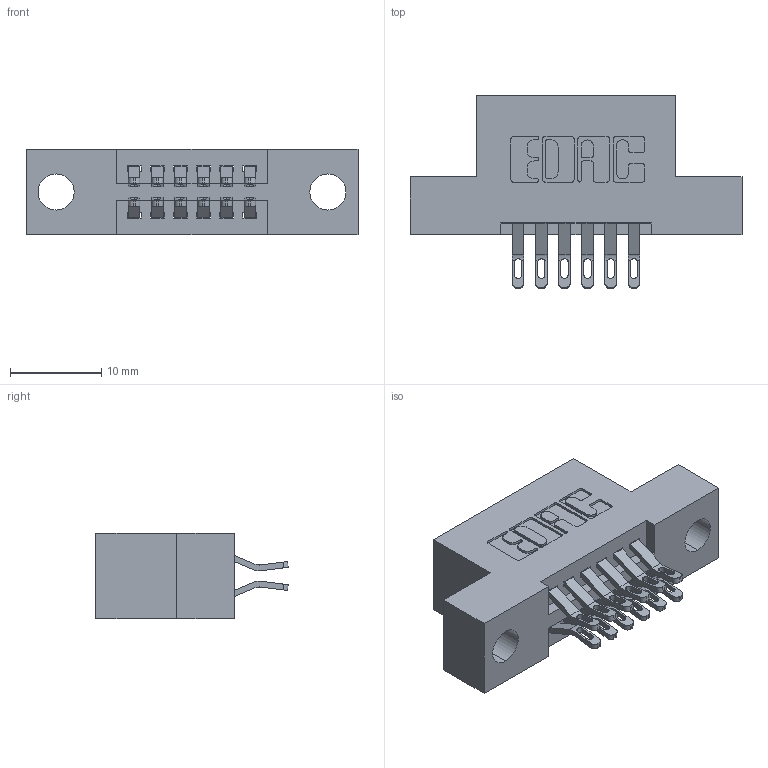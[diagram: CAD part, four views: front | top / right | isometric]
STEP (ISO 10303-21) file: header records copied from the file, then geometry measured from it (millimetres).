
FILE_DESCRIPTION (( 'STEP AP203' ), '1' );
FILE_NAME ('345-012-555-204.STEP', '2021-05-19T15:48:22', ( '' ), ( '' ), 'SwSTEP 2.0', 'SolidWorks 2020', '' );
FILE_SCHEMA (( 'CONFIG_CONTROL_DESIGN' ));
Length unit declared in the file: inch
Products named in the file (3): 345-012-555-204; 345-292-001_555 Tail; 345 Part_Flush Mounting Lugs - 0.156 Dia-TI
Assembly tree (13 placements, depth 2):
  345-012-555-204
    345 Part_Flush Mounting Lugs - 0.156 Dia-TI
    345-292-001_555 Tail  x12
Bounding box: 36.45 x 21.13 x 9.4 mm (x, y, z)
Volume: 3135.4 mm3; surface area: 3910 mm2
Topology: 13 solids, 13 shells, 812 faces, 2501 edges, 1666 vertices
Faces by surface type: plane 466, cylinder 346
Entity records: 10299 total; most frequent: CARTESIAN_POINT 1800, ORIENTED_EDGE 1702, DIRECTION 1599, EDGE_CURVE 851, LINE 675, VECTOR 675, VERTEX_POINT 566, AXIS2_PLACEMENT_3D 462
